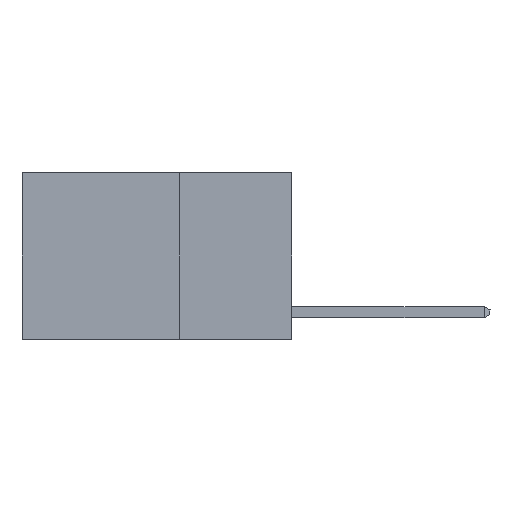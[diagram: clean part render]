
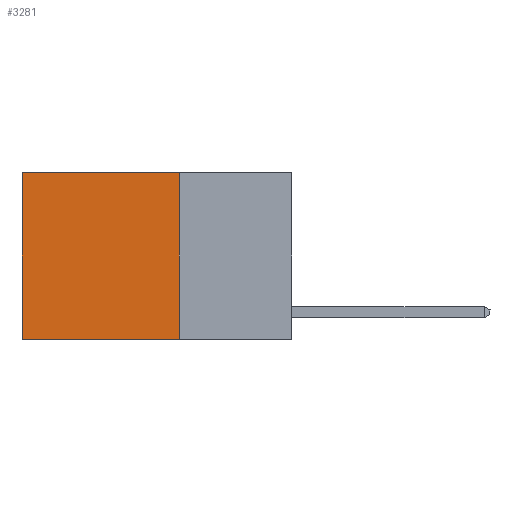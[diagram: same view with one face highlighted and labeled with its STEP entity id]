
A CAD part, left-side view. The second image highlights one B-rep face of the part: STEP entity #3281.
In plain terms, the highlighted planar face has unit normal (-1, 0, 0).
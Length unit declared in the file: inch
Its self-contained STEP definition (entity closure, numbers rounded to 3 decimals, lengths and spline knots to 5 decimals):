
#23 = LINE ( 'NONE', #9203, #6564 ) ;
#1531 = EDGE_CURVE ( 'NONE', #3935, #5784, #2196, .T. ) ;
#1587 = VECTOR ( 'NONE', #9040, 39.37008 ) ;
#2005 = CARTESIAN_POINT ( 'NONE',  ( 0.2625, 0.25, 0. ) ) ;
#2190 = EDGE_CURVE ( 'NONE', #8985, #8946, #7770, .T. ) ;
#2196 = LINE ( 'NONE', #5097, #6618 ) ;
#2315 = CARTESIAN_POINT ( 'NONE',  ( 0.2625, 0.25, 0. ) ) ;
#3039 = AXIS2_PLACEMENT_3D ( 'NONE', #2005, #7975, #5436 ) ;
#3085 = ORIENTED_EDGE ( 'NONE', *, *, #2190, .T. ) ;
#3281 = ADVANCED_FACE ( 'NONE', ( #8417 ), #4438, .F. ) ;
#3488 = EDGE_CURVE ( 'NONE', #3935, #8985, #23, .T. ) ;
#3935 = VERTEX_POINT ( 'NONE', #2315 ) ;
#4189 = DIRECTION ( 'NONE',  ( 0., 0., -1. ) ) ;
#4438 = PLANE ( 'NONE',  #3039 ) ;
#4481 = EDGE_CURVE ( 'NONE', #5784, #8946, #9207, .T. ) ;
#4826 = DIRECTION ( 'NONE',  ( 0., 1., 0. ) ) ;
#4901 = CARTESIAN_POINT ( 'NONE',  ( 0.2625, 0.6, -0.37 ) ) ;
#5097 = CARTESIAN_POINT ( 'NONE',  ( 0.2625, 0.25, 0. ) ) ;
#5208 = CARTESIAN_POINT ( 'NONE',  ( 0.2625, 0.25, -0.37 ) ) ;
#5436 = DIRECTION ( 'NONE',  ( 0., 0., -1. ) ) ;
#5784 = VERTEX_POINT ( 'NONE', #5208 ) ;
#5970 = EDGE_LOOP ( 'NONE', ( #3085, #10177, #7410, #9169 ) ) ;
#6564 = VECTOR ( 'NONE', #4826, 39.37008 ) ;
#6579 = CARTESIAN_POINT ( 'NONE',  ( 0.2625, 0.25, -0.37 ) ) ;
#6618 = VECTOR ( 'NONE', #4189, 39.37008 ) ;
#6694 = CARTESIAN_POINT ( 'NONE',  ( 0.2625, 0.6, 0. ) ) ;
#7410 = ORIENTED_EDGE ( 'NONE', *, *, #1531, .F. ) ;
#7770 = LINE ( 'NONE', #6694, #9644 ) ;
#7975 = DIRECTION ( 'NONE',  ( 1., 0., 0. ) ) ;
#8417 = FACE_OUTER_BOUND ( 'NONE', #5970, .T. ) ;
#8946 = VERTEX_POINT ( 'NONE', #4901 ) ;
#8985 = VERTEX_POINT ( 'NONE', #10760 ) ;
#9040 = DIRECTION ( 'NONE',  ( 0., 1., 0. ) ) ;
#9169 = ORIENTED_EDGE ( 'NONE', *, *, #3488, .T. ) ;
#9203 = CARTESIAN_POINT ( 'NONE',  ( 0.2625, 0.25, 0. ) ) ;
#9207 = LINE ( 'NONE', #6579, #1587 ) ;
#9232 = DIRECTION ( 'NONE',  ( 0., 0., -1. ) ) ;
#9644 = VECTOR ( 'NONE', #9232, 39.37008 ) ;
#10177 = ORIENTED_EDGE ( 'NONE', *, *, #4481, .F. ) ;
#10760 = CARTESIAN_POINT ( 'NONE',  ( 0.2625, 0.6, 0. ) ) ;
